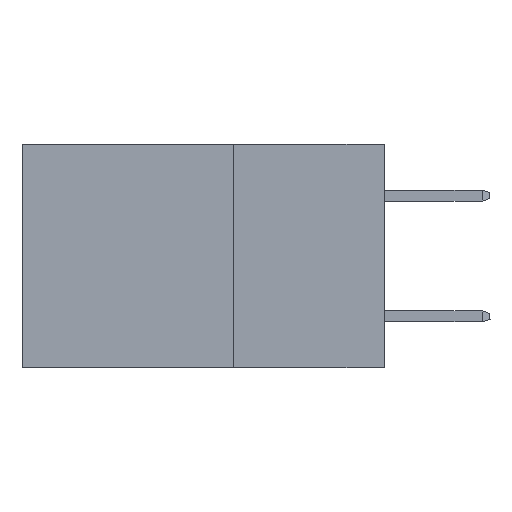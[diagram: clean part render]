
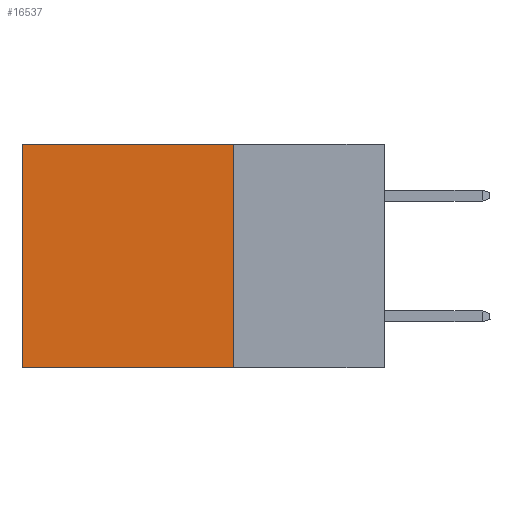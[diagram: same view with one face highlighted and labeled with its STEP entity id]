
A CAD part, left-side view. The second image highlights one B-rep face of the part: STEP entity #16537.
In plain terms, the highlighted planar face has unit normal (-1, 0, 0).
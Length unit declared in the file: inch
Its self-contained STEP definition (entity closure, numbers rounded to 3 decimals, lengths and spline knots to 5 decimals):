
#1442 = VERTEX_POINT ( 'NONE', #16705 ) ;
#1578 = ORIENTED_EDGE ( 'NONE', *, *, #7186, .T. ) ;
#2334 = LINE ( 'NONE', #4122, #15771 ) ;
#2445 = LINE ( 'NONE', #12348, #15881 ) ;
#3788 = FACE_OUTER_BOUND ( 'NONE', #16203, .T. ) ;
#3935 = PLANE ( 'NONE',  #11688 ) ;
#4122 = CARTESIAN_POINT ( 'NONE',  ( 0.2615, 0.25, -0.37 ) ) ;
#4242 = DIRECTION ( 'NONE',  ( 0., 0., -1. ) ) ;
#4729 = VERTEX_POINT ( 'NONE', #11574 ) ;
#5119 = DIRECTION ( 'NONE',  ( 0., 1., 0. ) ) ;
#5687 = CARTESIAN_POINT ( 'NONE',  ( 0.2615, 0.25, -0.37 ) ) ;
#5706 = DIRECTION ( 'NONE',  ( 0., 1., 0. ) ) ;
#6596 = ORIENTED_EDGE ( 'NONE', *, *, #10349, .F. ) ;
#6653 = DIRECTION ( 'NONE',  ( 0., 0., -1. ) ) ;
#7186 = EDGE_CURVE ( 'NONE', #9749, #1442, #2445, .T. ) ;
#7754 = CARTESIAN_POINT ( 'NONE',  ( 0.2615, 0.25, 0. ) ) ;
#7762 = EDGE_CURVE ( 'NONE', #4729, #1442, #14652, .T. ) ;
#8352 = ORIENTED_EDGE ( 'NONE', *, *, #7762, .F. ) ;
#8354 = CARTESIAN_POINT ( 'NONE',  ( 0.2615, 0.6, 0. ) ) ;
#9477 = LINE ( 'NONE', #7754, #15349 ) ;
#9749 = VERTEX_POINT ( 'NONE', #8354 ) ;
#9977 = ORIENTED_EDGE ( 'NONE', *, *, #16456, .T. ) ;
#10349 = EDGE_CURVE ( 'NONE', #11454, #4729, #2334, .T. ) ;
#11454 = VERTEX_POINT ( 'NONE', #13092 ) ;
#11574 = CARTESIAN_POINT ( 'NONE',  ( 0.2615, 0.25, -0.37 ) ) ;
#11688 = AXIS2_PLACEMENT_3D ( 'NONE', #13352, #14679, #6653 ) ;
#12228 = DIRECTION ( 'NONE',  ( 0., 0., -1. ) ) ;
#12348 = CARTESIAN_POINT ( 'NONE',  ( 0.2615, 0.6, -0.37 ) ) ;
#13092 = CARTESIAN_POINT ( 'NONE',  ( 0.2615, 0.25, 0. ) ) ;
#13352 = CARTESIAN_POINT ( 'NONE',  ( 0.2615, 0.25, -0.37 ) ) ;
#13818 = VECTOR ( 'NONE', #5706, 39.37008 ) ;
#14652 = LINE ( 'NONE', #5687, #13818 ) ;
#14679 = DIRECTION ( 'NONE',  ( 1., 0., 0. ) ) ;
#15349 = VECTOR ( 'NONE', #5119, 39.37008 ) ;
#15771 = VECTOR ( 'NONE', #4242, 39.37008 ) ;
#15881 = VECTOR ( 'NONE', #12228, 39.37008 ) ;
#16203 = EDGE_LOOP ( 'NONE', ( #1578, #8352, #6596, #9977 ) ) ;
#16456 = EDGE_CURVE ( 'NONE', #11454, #9749, #9477, .T. ) ;
#16537 = ADVANCED_FACE ( 'NONE', ( #3788 ), #3935, .F. ) ;
#16705 = CARTESIAN_POINT ( 'NONE',  ( 0.2615, 0.6, -0.37 ) ) ;
